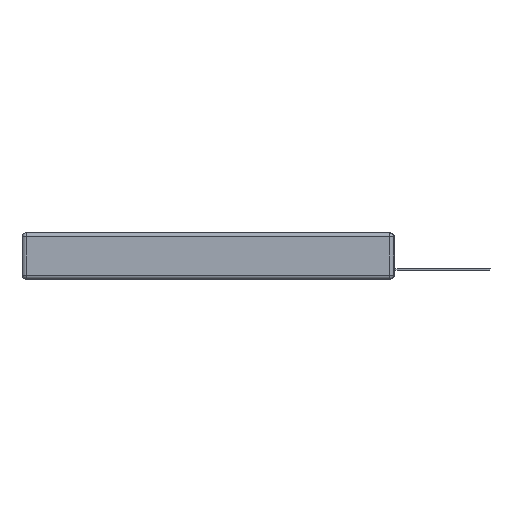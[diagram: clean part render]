
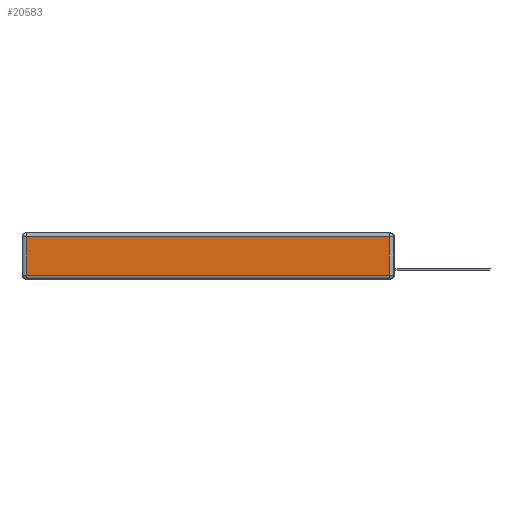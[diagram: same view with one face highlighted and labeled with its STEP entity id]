
A CAD part, left-side view. The second image highlights one B-rep face of the part: STEP entity #20583.
In plain terms, the highlighted planar face has unit normal (-1, 0, 0).
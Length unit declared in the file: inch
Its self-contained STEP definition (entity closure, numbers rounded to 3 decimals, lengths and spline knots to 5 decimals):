
#768 = EDGE_CURVE ( 'NONE', #13822, #2985, #20852, .T. ) ;
#2712 = LINE ( 'NONE', #16384, #9819 ) ;
#2985 = VERTEX_POINT ( 'NONE', #13567 ) ;
#3668 = VERTEX_POINT ( 'NONE', #14179 ) ;
#5628 = EDGE_LOOP ( 'NONE', ( #5739, #7562, #9220, #11876 ) ) ;
#5739 = ORIENTED_EDGE ( 'NONE', *, *, #11777, .T. ) ;
#5867 = CARTESIAN_POINT ( 'NONE',  ( 0., 0.03, -0.343 ) ) ;
#7562 = ORIENTED_EDGE ( 'NONE', *, *, #20084, .T. ) ;
#8004 = VECTOR ( 'NONE', #19859, 39.37008 ) ;
#9079 = LINE ( 'NONE', #19940, #8004 ) ;
#9220 = ORIENTED_EDGE ( 'NONE', *, *, #16585, .T. ) ;
#9619 = FACE_OUTER_BOUND ( 'NONE', #5628, .T. ) ;
#9819 = VECTOR ( 'NONE', #19504, 39.37008 ) ;
#9962 = VECTOR ( 'NONE', #20499, 39.37008 ) ;
#10222 = CARTESIAN_POINT ( 'NONE',  ( 0., 0., -0.343 ) ) ;
#11158 = DIRECTION ( 'NONE',  ( 0., 0., 1. ) ) ;
#11777 = EDGE_CURVE ( 'NONE', #2985, #13435, #2712, .T. ) ;
#11876 = ORIENTED_EDGE ( 'NONE', *, *, #768, .T. ) ;
#13372 = VECTOR ( 'NONE', #11158, 39.37008 ) ;
#13435 = VERTEX_POINT ( 'NONE', #13874 ) ;
#13567 = CARTESIAN_POINT ( 'NONE',  ( 0., 2.72, -0.313 ) ) ;
#13573 = AXIS2_PLACEMENT_3D ( 'NONE', #10222, #17087, #18569 ) ;
#13822 = VERTEX_POINT ( 'NONE', #15271 ) ;
#13874 = CARTESIAN_POINT ( 'NONE',  ( 0., 0.03, -0.313 ) ) ;
#14179 = CARTESIAN_POINT ( 'NONE',  ( 0., 0.03, -0.03 ) ) ;
#14188 = LINE ( 'NONE', #5867, #13372 ) ;
#15145 = PLANE ( 'NONE',  #13573 ) ;
#15271 = CARTESIAN_POINT ( 'NONE',  ( 0., 2.72, -0.03 ) ) ;
#16384 = CARTESIAN_POINT ( 'NONE',  ( 0., 0., -0.313 ) ) ;
#16585 = EDGE_CURVE ( 'NONE', #3668, #13822, #9079, .T. ) ;
#16963 = CARTESIAN_POINT ( 'NONE',  ( 0., 2.72, -0.343 ) ) ;
#17087 = DIRECTION ( 'NONE',  ( -1., 0., 0. ) ) ;
#18569 = DIRECTION ( 'NONE',  ( 0., 0., 1. ) ) ;
#19504 = DIRECTION ( 'NONE',  ( 0., -1., 0. ) ) ;
#19859 = DIRECTION ( 'NONE',  ( 0., 1., 0. ) ) ;
#19940 = CARTESIAN_POINT ( 'NONE',  ( 0., 2.75, -0.03 ) ) ;
#20084 = EDGE_CURVE ( 'NONE', #13435, #3668, #14188, .T. ) ;
#20499 = DIRECTION ( 'NONE',  ( 0., 0., -1. ) ) ;
#20583 = ADVANCED_FACE ( 'NONE', ( #9619 ), #15145, .T. ) ;
#20852 = LINE ( 'NONE', #16963, #9962 ) ;
